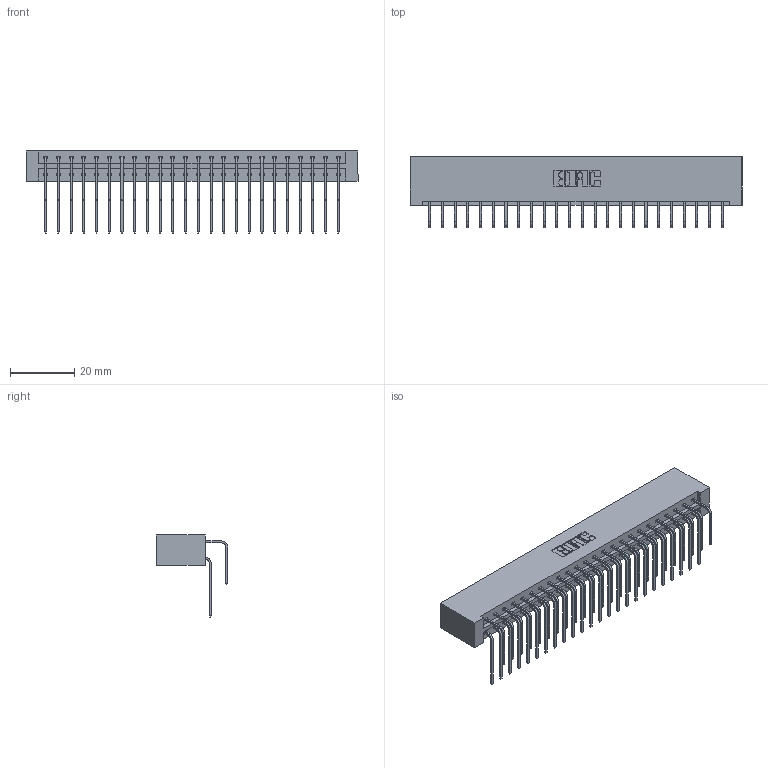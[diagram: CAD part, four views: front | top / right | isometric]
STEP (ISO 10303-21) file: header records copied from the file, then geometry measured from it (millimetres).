
FILE_DESCRIPTION (( 'STEP AP203' ), '1' );
FILE_NAME ('833-048-558-201.STEP', '2020-06-04T16:32:03', ( '' ), ( '' ), 'SwSTEP 2.0', 'SolidWorks 2020', '' );
FILE_SCHEMA (( 'CONFIG_CONTROL_DESIGN' ));
Length unit declared in the file: inch
Products named in the file (4): 833-048-558-201; 833 Part_Lugless; 345-292-001_558 559 Tail - 1; 345-292-001_558 Tail - 2
Assembly tree (49 placements, depth 2):
  833-048-558-201
    833 Part_Lugless
    345-292-001_558 559 Tail - 1  x24
    345-292-001_558 Tail - 2  x24
Bounding box: 103.35 x 22.17 x 25.53 mm (x, y, z)
Volume: 11292.5 mm3; surface area: 14560.7 mm2
Topology: 49 solids, 49 shells, 2698 faces, 8015 edges, 5278 vertices
Faces by surface type: plane 1890, cylinder 808
Entity records: 19275 total; most frequent: CARTESIAN_POINT 3265, ORIENTED_EDGE 3150, DIRECTION 2795, EDGE_CURVE 1575, LINE 1415, VECTOR 1415, VERTEX_POINT 1046, AXIS2_PLACEMENT_3D 690
